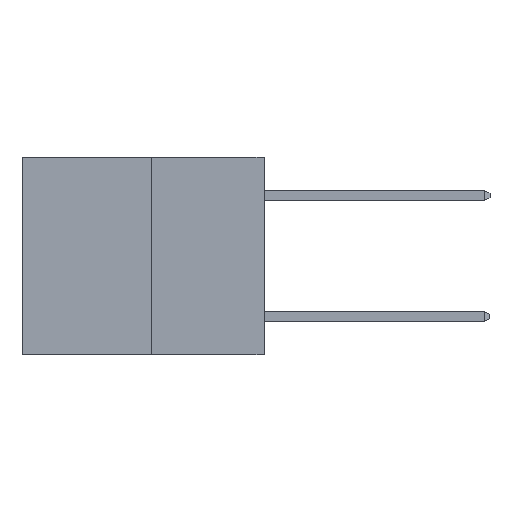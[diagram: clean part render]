
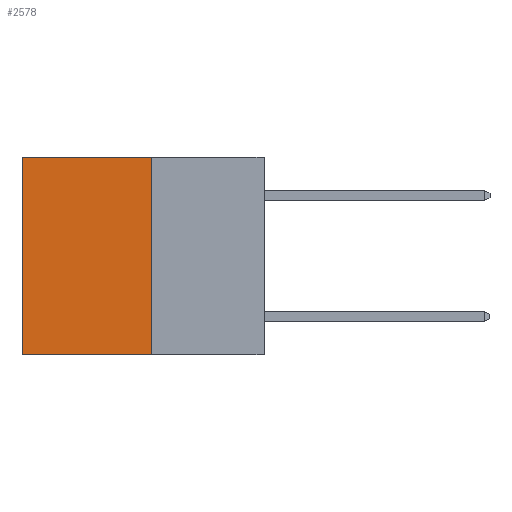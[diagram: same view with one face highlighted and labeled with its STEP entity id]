
A CAD part, left-side view. The second image highlights one B-rep face of the part: STEP entity #2578.
In plain terms, the highlighted planar face has unit normal (-1, 0, 0).
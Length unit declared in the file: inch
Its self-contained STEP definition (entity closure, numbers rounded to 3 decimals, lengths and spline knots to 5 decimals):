
#565 = DIRECTION ( 'NONE',  ( 0., 0., -1. ) ) ;
#722 = CARTESIAN_POINT ( 'NONE',  ( 0.3165, 0.28, 0. ) ) ;
#1641 = ORIENTED_EDGE ( 'NONE', *, *, #13923, .T. ) ;
#1770 = VECTOR ( 'NONE', #5690, 39.37008 ) ;
#2578 = ADVANCED_FACE ( 'NONE', ( #6133 ), #9916, .F. ) ;
#3220 = VERTEX_POINT ( 'NONE', #4085 ) ;
#3395 = CARTESIAN_POINT ( 'NONE',  ( 0.3165, 0.28, -0.49 ) ) ;
#4059 = EDGE_CURVE ( 'NONE', #9997, #10691, #9191, .T. ) ;
#4085 = CARTESIAN_POINT ( 'NONE',  ( 0.3165, 0.28, 0. ) ) ;
#4934 = DIRECTION ( 'NONE',  ( 0., 1., 0. ) ) ;
#5690 = DIRECTION ( 'NONE',  ( 0., 0., -1. ) ) ;
#6133 = FACE_OUTER_BOUND ( 'NONE', #14726, .T. ) ;
#6279 = VECTOR ( 'NONE', #4934, 39.37008 ) ;
#7035 = ORIENTED_EDGE ( 'NONE', *, *, #8564, .T. ) ;
#7252 = CARTESIAN_POINT ( 'NONE',  ( 0.3165, 0.28, -0.49 ) ) ;
#7419 = DIRECTION ( 'NONE',  ( 0., 0., -1. ) ) ;
#8423 = VECTOR ( 'NONE', #7419, 39.37008 ) ;
#8465 = CARTESIAN_POINT ( 'NONE',  ( 0.3165, 0.28, -0.49 ) ) ;
#8564 = EDGE_CURVE ( 'NONE', #3220, #10130, #11266, .T. ) ;
#8809 = DIRECTION ( 'NONE',  ( 1., 0., 0. ) ) ;
#8964 = DIRECTION ( 'NONE',  ( 0., 1., 0. ) ) ;
#9191 = LINE ( 'NONE', #8465, #6279 ) ;
#9916 = PLANE ( 'NONE',  #12528 ) ;
#9997 = VERTEX_POINT ( 'NONE', #7252 ) ;
#10130 = VERTEX_POINT ( 'NONE', #13493 ) ;
#10691 = VERTEX_POINT ( 'NONE', #10880 ) ;
#10880 = CARTESIAN_POINT ( 'NONE',  ( 0.3165, 0.6, -0.49 ) ) ;
#11266 = LINE ( 'NONE', #722, #13813 ) ;
#11555 = LINE ( 'NONE', #12216, #8423 ) ;
#12216 = CARTESIAN_POINT ( 'NONE',  ( 0.3165, 0.6, -0.49 ) ) ;
#12528 = AXIS2_PLACEMENT_3D ( 'NONE', #13393, #8809, #565 ) ;
#12722 = ORIENTED_EDGE ( 'NONE', *, *, #4059, .F. ) ;
#13393 = CARTESIAN_POINT ( 'NONE',  ( 0.3165, 0.28, -0.49 ) ) ;
#13493 = CARTESIAN_POINT ( 'NONE',  ( 0.3165, 0.6, 0. ) ) ;
#13813 = VECTOR ( 'NONE', #8964, 39.37008 ) ;
#13910 = LINE ( 'NONE', #3395, #1770 ) ;
#13923 = EDGE_CURVE ( 'NONE', #10130, #10691, #11555, .T. ) ;
#13962 = ORIENTED_EDGE ( 'NONE', *, *, #14078, .F. ) ;
#14078 = EDGE_CURVE ( 'NONE', #3220, #9997, #13910, .T. ) ;
#14726 = EDGE_LOOP ( 'NONE', ( #1641, #12722, #13962, #7035 ) ) ;
